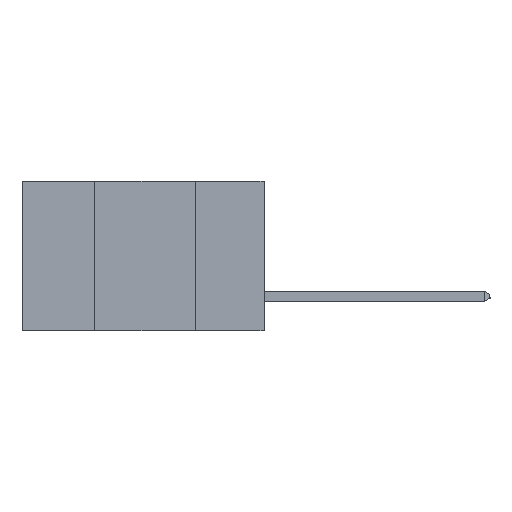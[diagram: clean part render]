
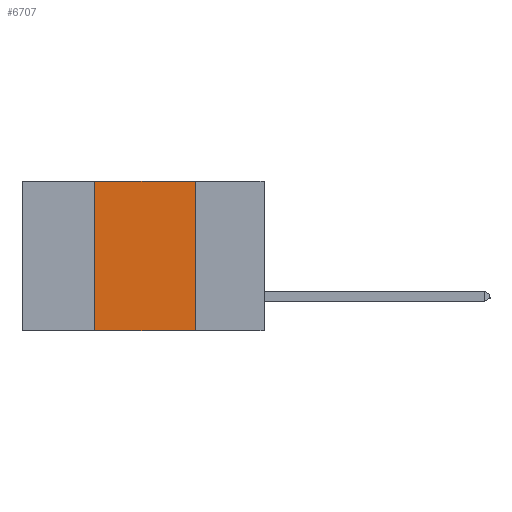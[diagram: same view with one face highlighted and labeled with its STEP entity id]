
A CAD part, left-side view. The second image highlights one B-rep face of the part: STEP entity #6707.
In plain terms, the highlighted planar face has unit normal (-1, 0, 0).
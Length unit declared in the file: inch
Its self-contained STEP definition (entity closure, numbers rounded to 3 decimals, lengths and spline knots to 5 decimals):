
#88 = LINE ( 'NONE', #4303, #10327 ) ;
#540 = DIRECTION ( 'NONE',  ( 0., 0., -1. ) ) ;
#543 = LINE ( 'NONE', #5182, #4505 ) ;
#2153 = VECTOR ( 'NONE', #7801, 39.37008 ) ;
#2670 = VECTOR ( 'NONE', #7752, 39.37008 ) ;
#3133 = ORIENTED_EDGE ( 'NONE', *, *, #10201, .F. ) ;
#3156 = VERTEX_POINT ( 'NONE', #3172 ) ;
#3172 = CARTESIAN_POINT ( 'NONE',  ( 0., 0.42, 0. ) ) ;
#3640 = VERTEX_POINT ( 'NONE', #4650 ) ;
#4303 = CARTESIAN_POINT ( 'NONE',  ( 0., 0.17, 0. ) ) ;
#4505 = VECTOR ( 'NONE', #6034, 39.37008 ) ;
#4650 = CARTESIAN_POINT ( 'NONE',  ( 0., 0.42, -0.37 ) ) ;
#4973 = VERTEX_POINT ( 'NONE', #10398 ) ;
#5125 = DIRECTION ( 'NONE',  ( 0., 0., -1. ) ) ;
#5182 = CARTESIAN_POINT ( 'NONE',  ( 0., 0.6, -0.37 ) ) ;
#5577 = DIRECTION ( 'NONE',  ( 1., 0., 0. ) ) ;
#6034 = DIRECTION ( 'NONE',  ( 0., -1., 0. ) ) ;
#6505 = EDGE_CURVE ( 'NONE', #3156, #4973, #9400, .T. ) ;
#6707 = ADVANCED_FACE ( 'NONE', ( #9522 ), #10241, .F. ) ;
#6781 = ORIENTED_EDGE ( 'NONE', *, *, #10026, .F. ) ;
#6986 = CARTESIAN_POINT ( 'NONE',  ( 0., 0.6, 0. ) ) ;
#7033 = CARTESIAN_POINT ( 'NONE',  ( 0., 0.42, 0. ) ) ;
#7206 = EDGE_CURVE ( 'NONE', #3640, #7697, #543, .T. ) ;
#7679 = AXIS2_PLACEMENT_3D ( 'NONE', #8758, #5577, #540 ) ;
#7697 = VERTEX_POINT ( 'NONE', #8995 ) ;
#7752 = DIRECTION ( 'NONE',  ( 0., -1., 0. ) ) ;
#7801 = DIRECTION ( 'NONE',  ( 0., 0., 1. ) ) ;
#8451 = LINE ( 'NONE', #7033, #2153 ) ;
#8758 = CARTESIAN_POINT ( 'NONE',  ( 0., 0.6, 0. ) ) ;
#8995 = CARTESIAN_POINT ( 'NONE',  ( 0., 0.17, -0.37 ) ) ;
#9090 = ORIENTED_EDGE ( 'NONE', *, *, #6505, .F. ) ;
#9400 = LINE ( 'NONE', #6986, #2670 ) ;
#9522 = FACE_OUTER_BOUND ( 'NONE', #9892, .T. ) ;
#9567 = ORIENTED_EDGE ( 'NONE', *, *, #7206, .T. ) ;
#9892 = EDGE_LOOP ( 'NONE', ( #6781, #9090, #3133, #9567 ) ) ;
#10026 = EDGE_CURVE ( 'NONE', #4973, #7697, #88, .T. ) ;
#10201 = EDGE_CURVE ( 'NONE', #3640, #3156, #8451, .T. ) ;
#10241 = PLANE ( 'NONE',  #7679 ) ;
#10327 = VECTOR ( 'NONE', #5125, 39.37008 ) ;
#10398 = CARTESIAN_POINT ( 'NONE',  ( 0., 0.17, 0. ) ) ;
